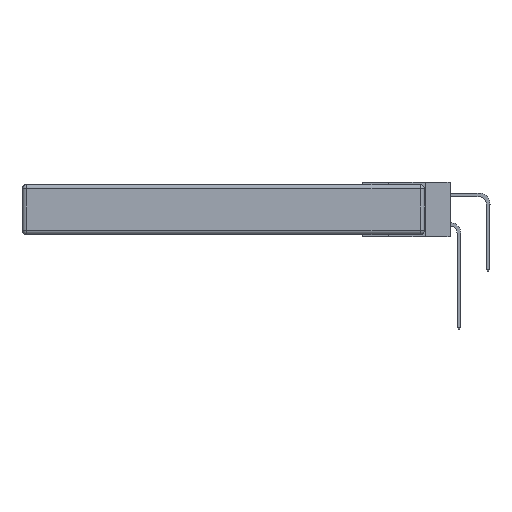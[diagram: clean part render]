
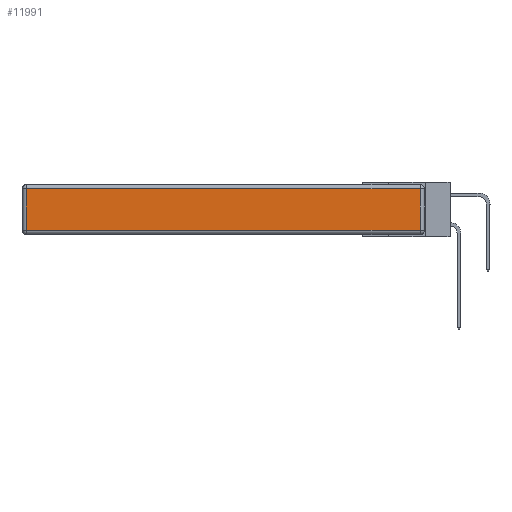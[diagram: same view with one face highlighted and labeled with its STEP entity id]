
A CAD part, left-side view. The second image highlights one B-rep face of the part: STEP entity #11991.
In plain terms, the highlighted planar face has unit normal (-1, 0, 0).
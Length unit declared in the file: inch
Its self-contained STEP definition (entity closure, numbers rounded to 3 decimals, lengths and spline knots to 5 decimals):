
#395 = CARTESIAN_POINT ( 'NONE',  ( 0., 0., -0.313 ) ) ;
#664 = VECTOR ( 'NONE', #18750, 39.37008 ) ;
#2518 = CARTESIAN_POINT ( 'NONE',  ( 0., 2.72, -0.03 ) ) ;
#3224 = ORIENTED_EDGE ( 'NONE', *, *, #25805, .T. ) ;
#3571 = DIRECTION ( 'NONE',  ( 0., 0., -1. ) ) ;
#5373 = CARTESIAN_POINT ( 'NONE',  ( 0., 0.03, -0.343 ) ) ;
#5850 = ORIENTED_EDGE ( 'NONE', *, *, #29878, .T. ) ;
#6670 = EDGE_CURVE ( 'NONE', #31664, #22092, #18093, .T. ) ;
#6743 = EDGE_LOOP ( 'NONE', ( #32155, #3224, #5850, #9321 ) ) ;
#7437 = CARTESIAN_POINT ( 'NONE',  ( 0., 2.75, -0.03 ) ) ;
#9321 = ORIENTED_EDGE ( 'NONE', *, *, #15421, .T. ) ;
#9538 = CARTESIAN_POINT ( 'NONE',  ( 0., 2.72, -0.313 ) ) ;
#10146 = CARTESIAN_POINT ( 'NONE',  ( 0., 2.72, -0.343 ) ) ;
#11194 = CARTESIAN_POINT ( 'NONE',  ( 0., 0.03, -0.313 ) ) ;
#11991 = ADVANCED_FACE ( 'NONE', ( #23839 ), #28252, .T. ) ;
#12652 = VECTOR ( 'NONE', #20097, 39.37008 ) ;
#12922 = DIRECTION ( 'NONE',  ( -1., 0., 0. ) ) ;
#15421 = EDGE_CURVE ( 'NONE', #27006, #31664, #26073, .T. ) ;
#17538 = VERTEX_POINT ( 'NONE', #28910 ) ;
#18093 = LINE ( 'NONE', #395, #664 ) ;
#18750 = DIRECTION ( 'NONE',  ( 0., -1., 0. ) ) ;
#19294 = VECTOR ( 'NONE', #3571, 39.37008 ) ;
#20097 = DIRECTION ( 'NONE',  ( 0., 1., 0. ) ) ;
#20237 = LINE ( 'NONE', #5373, #25010 ) ;
#20298 = AXIS2_PLACEMENT_3D ( 'NONE', #32936, #12922, #30478 ) ;
#20739 = DIRECTION ( 'NONE',  ( 0., 0., 1. ) ) ;
#22092 = VERTEX_POINT ( 'NONE', #11194 ) ;
#23839 = FACE_OUTER_BOUND ( 'NONE', #6743, .T. ) ;
#25010 = VECTOR ( 'NONE', #20739, 39.37008 ) ;
#25805 = EDGE_CURVE ( 'NONE', #22092, #17538, #20237, .T. ) ;
#26073 = LINE ( 'NONE', #10146, #19294 ) ;
#26341 = LINE ( 'NONE', #7437, #12652 ) ;
#27006 = VERTEX_POINT ( 'NONE', #2518 ) ;
#28252 = PLANE ( 'NONE',  #20298 ) ;
#28910 = CARTESIAN_POINT ( 'NONE',  ( 0., 0.03, -0.03 ) ) ;
#29878 = EDGE_CURVE ( 'NONE', #17538, #27006, #26341, .T. ) ;
#30478 = DIRECTION ( 'NONE',  ( 0., 0., 1. ) ) ;
#31664 = VERTEX_POINT ( 'NONE', #9538 ) ;
#32155 = ORIENTED_EDGE ( 'NONE', *, *, #6670, .T. ) ;
#32936 = CARTESIAN_POINT ( 'NONE',  ( 0., 0., -0.343 ) ) ;
